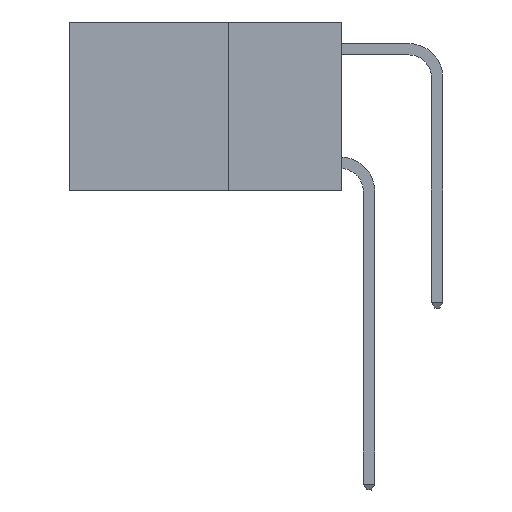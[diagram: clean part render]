
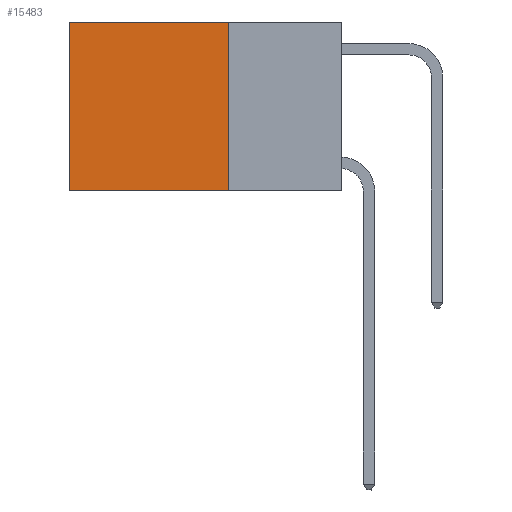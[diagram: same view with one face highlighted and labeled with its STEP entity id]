
A CAD part, left-side view. The second image highlights one B-rep face of the part: STEP entity #15483.
In plain terms, the highlighted planar face has unit normal (-1, 0, 0).
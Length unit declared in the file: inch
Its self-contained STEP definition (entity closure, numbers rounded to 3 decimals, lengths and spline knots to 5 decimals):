
#652 = PLANE ( 'NONE',  #17462 ) ;
#777 = DIRECTION ( 'NONE',  ( 1., 0., 0. ) ) ;
#1135 = VECTOR ( 'NONE', #20175, 39.37008 ) ;
#1521 = CARTESIAN_POINT ( 'NONE',  ( 0.2625, 0.6, 0. ) ) ;
#1664 = EDGE_CURVE ( 'NONE', #5043, #16853, #24583, .T. ) ;
#1701 = LINE ( 'NONE', #21288, #7098 ) ;
#2131 = ORIENTED_EDGE ( 'NONE', *, *, #20878, .F. ) ;
#2831 = CARTESIAN_POINT ( 'NONE',  ( 0.2625, 0.6, -0.37 ) ) ;
#4252 = ORIENTED_EDGE ( 'NONE', *, *, #1664, .T. ) ;
#5043 = VERTEX_POINT ( 'NONE', #1521 ) ;
#5977 = LINE ( 'NONE', #23956, #1135 ) ;
#6001 = EDGE_CURVE ( 'NONE', #14576, #16853, #1701, .T. ) ;
#6524 = CARTESIAN_POINT ( 'NONE',  ( 0.2625, 0.25, 0. ) ) ;
#7098 = VECTOR ( 'NONE', #17285, 39.37008 ) ;
#8269 = ORIENTED_EDGE ( 'NONE', *, *, #6001, .F. ) ;
#10990 = LINE ( 'NONE', #15133, #16370 ) ;
#11051 = VECTOR ( 'NONE', #22757, 39.37008 ) ;
#12672 = DIRECTION ( 'NONE',  ( 0., 1., 0. ) ) ;
#12744 = ORIENTED_EDGE ( 'NONE', *, *, #25186, .T. ) ;
#14268 = CARTESIAN_POINT ( 'NONE',  ( 0.2625, 0.25, -0.37 ) ) ;
#14576 = VERTEX_POINT ( 'NONE', #14268 ) ;
#14746 = CARTESIAN_POINT ( 'NONE',  ( 0.2625, 0.6, 0. ) ) ;
#15133 = CARTESIAN_POINT ( 'NONE',  ( 0.2625, 0.25, 0. ) ) ;
#15483 = ADVANCED_FACE ( 'NONE', ( #16122 ), #652, .F. ) ;
#16122 = FACE_OUTER_BOUND ( 'NONE', #21172, .T. ) ;
#16370 = VECTOR ( 'NONE', #12672, 39.37008 ) ;
#16853 = VERTEX_POINT ( 'NONE', #2831 ) ;
#17285 = DIRECTION ( 'NONE',  ( 0., 1., 0. ) ) ;
#17462 = AXIS2_PLACEMENT_3D ( 'NONE', #20001, #777, #17924 ) ;
#17924 = DIRECTION ( 'NONE',  ( 0., 0., -1. ) ) ;
#20001 = CARTESIAN_POINT ( 'NONE',  ( 0.2625, 0.25, 0. ) ) ;
#20175 = DIRECTION ( 'NONE',  ( 0., 0., -1. ) ) ;
#20878 = EDGE_CURVE ( 'NONE', #23222, #14576, #5977, .T. ) ;
#21172 = EDGE_LOOP ( 'NONE', ( #4252, #8269, #2131, #12744 ) ) ;
#21288 = CARTESIAN_POINT ( 'NONE',  ( 0.2625, 0.25, -0.37 ) ) ;
#22757 = DIRECTION ( 'NONE',  ( 0., 0., -1. ) ) ;
#23222 = VERTEX_POINT ( 'NONE', #6524 ) ;
#23956 = CARTESIAN_POINT ( 'NONE',  ( 0.2625, 0.25, 0. ) ) ;
#24583 = LINE ( 'NONE', #14746, #11051 ) ;
#25186 = EDGE_CURVE ( 'NONE', #23222, #5043, #10990, .T. ) ;
